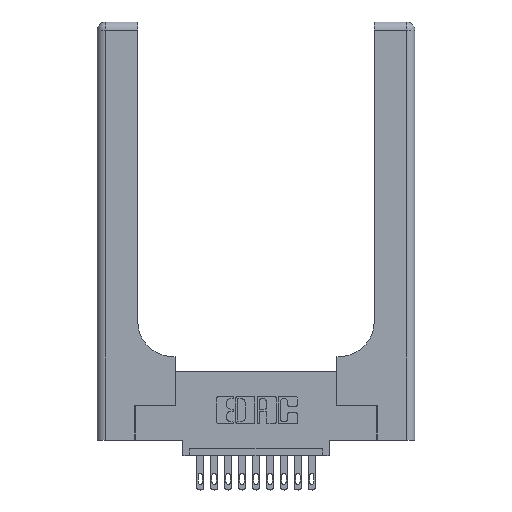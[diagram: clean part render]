
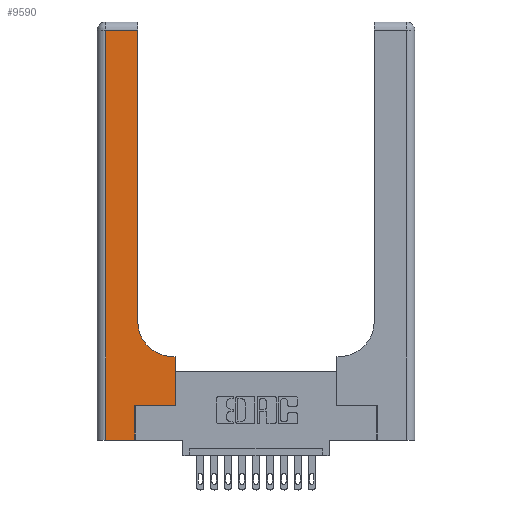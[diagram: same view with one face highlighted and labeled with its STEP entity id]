
A CAD part, top view. The second image highlights one B-rep face of the part: STEP entity #9590.
In plain terms, the highlighted planar face has unit normal (0, 0, 1).
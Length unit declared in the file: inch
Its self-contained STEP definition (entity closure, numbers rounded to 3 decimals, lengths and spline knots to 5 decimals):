
#40 = LINE ( 'NONE', #6423, #5369 ) ;
#183 = VERTEX_POINT ( 'NONE', #13133 ) ;
#448 = CARTESIAN_POINT ( 'NONE',  ( 0.06, 3., 0.37 ) ) ;
#511 = VERTEX_POINT ( 'NONE', #15085 ) ;
#565 = CARTESIAN_POINT ( 'NONE',  ( 0., 0., 0.37 ) ) ;
#735 = DIRECTION ( 'NONE',  ( 1., 0., 0. ) ) ;
#793 = EDGE_CURVE ( 'NONE', #9675, #12116, #40, .T. ) ;
#998 = CARTESIAN_POINT ( 'NONE',  ( 0., 2.94, 0.37 ) ) ;
#1002 = CARTESIAN_POINT ( 'NONE',  ( 0.5585, 0.25, 0.37 ) ) ;
#1090 = ORIENTED_EDGE ( 'NONE', *, *, #10468, .T. ) ;
#1092 = VECTOR ( 'NONE', #8857, 39.37008 ) ;
#1228 = CARTESIAN_POINT ( 'NONE',  ( 0.06, 0., 0.37 ) ) ;
#1243 = VERTEX_POINT ( 'NONE', #10867 ) ;
#2187 = VECTOR ( 'NONE', #735, 39.37008 ) ;
#2262 = CARTESIAN_POINT ( 'NONE',  ( 0.269, 0.25, 0.37 ) ) ;
#2326 = VECTOR ( 'NONE', #4971, 39.37008 ) ;
#2337 = DIRECTION ( 'NONE',  ( -1., 0., 0. ) ) ;
#2875 = CARTESIAN_POINT ( 'NONE',  ( 0.2915, 2.94, 0.37 ) ) ;
#3333 = ORIENTED_EDGE ( 'NONE', *, *, #13157, .T. ) ;
#3537 = DIRECTION ( 'NONE',  ( 0., 0., -1. ) ) ;
#3543 = EDGE_CURVE ( 'NONE', #9217, #9990, #8929, .T. ) ;
#4392 = ORIENTED_EDGE ( 'NONE', *, *, #7772, .T. ) ;
#4471 = CARTESIAN_POINT ( 'NONE',  ( 0., 3., 0.37 ) ) ;
#4577 = PLANE ( 'NONE',  #9491 ) ;
#4971 = DIRECTION ( 'NONE',  ( 0., 1., 0. ) ) ;
#4990 = ORIENTED_EDGE ( 'NONE', *, *, #11939, .T. ) ;
#4993 = CIRCLE ( 'NONE', #10254, 0.25 ) ;
#5369 = VECTOR ( 'NONE', #9749, 39.37008 ) ;
#5548 = LINE ( 'NONE', #998, #9497 ) ;
#5561 = LINE ( 'NONE', #565, #2187 ) ;
#5697 = LINE ( 'NONE', #1002, #2326 ) ;
#5817 = DIRECTION ( 'NONE',  ( 0., 0., -1. ) ) ;
#5955 = ORIENTED_EDGE ( 'NONE', *, *, #3543, .T. ) ;
#5991 = DIRECTION ( 'NONE',  ( -1., 0., 0. ) ) ;
#6092 = CARTESIAN_POINT ( 'NONE',  ( 0.269, 0., 0.37 ) ) ;
#6423 = CARTESIAN_POINT ( 'NONE',  ( 0.2915, 0.6, 0.37 ) ) ;
#6547 = CARTESIAN_POINT ( 'NONE',  ( 0.2915, 0.85, 0.37 ) ) ;
#6905 = CARTESIAN_POINT ( 'NONE',  ( 0.269, 0., 0.37 ) ) ;
#7039 = VERTEX_POINT ( 'NONE', #1228 ) ;
#7416 = LINE ( 'NONE', #448, #8202 ) ;
#7564 = VECTOR ( 'NONE', #13747, 39.37008 ) ;
#7772 = EDGE_CURVE ( 'NONE', #183, #1243, #8458, .T. ) ;
#7828 = FACE_OUTER_BOUND ( 'NONE', #9893, .T. ) ;
#8202 = VECTOR ( 'NONE', #10582, 39.37008 ) ;
#8458 = LINE ( 'NONE', #2262, #1092 ) ;
#8857 = DIRECTION ( 'NONE',  ( 1., 0., 0. ) ) ;
#8929 = LINE ( 'NONE', #15086, #7564 ) ;
#8968 = ORIENTED_EDGE ( 'NONE', *, *, #793, .T. ) ;
#9217 = VERTEX_POINT ( 'NONE', #6547 ) ;
#9491 = AXIS2_PLACEMENT_3D ( 'NONE', #4471, #5817, #5991 ) ;
#9497 = VECTOR ( 'NONE', #2337, 39.37008 ) ;
#9590 = ADVANCED_FACE ( 'NONE', ( #7828 ), #4577, .F. ) ;
#9675 = VERTEX_POINT ( 'NONE', #10587 ) ;
#9749 = DIRECTION ( 'NONE',  ( -1., 0., 0. ) ) ;
#9893 = EDGE_LOOP ( 'NONE', ( #5955, #3333, #1090, #14404, #4990, #4392, #12076, #8968, #10879 ) ) ;
#9896 = DIRECTION ( 'NONE',  ( 1., 0., 0. ) ) ;
#9950 = VECTOR ( 'NONE', #11904, 39.37008 ) ;
#9990 = VERTEX_POINT ( 'NONE', #2875 ) ;
#10254 = AXIS2_PLACEMENT_3D ( 'NONE', #12479, #3537, #9896 ) ;
#10468 = EDGE_CURVE ( 'NONE', #511, #7039, #7416, .T. ) ;
#10582 = DIRECTION ( 'NONE',  ( 0., -1., 0. ) ) ;
#10587 = CARTESIAN_POINT ( 'NONE',  ( 0.5585, 0.6, 0.37 ) ) ;
#10867 = CARTESIAN_POINT ( 'NONE',  ( 0.5585, 0.25, 0.37 ) ) ;
#10879 = ORIENTED_EDGE ( 'NONE', *, *, #10948, .T. ) ;
#10948 = EDGE_CURVE ( 'NONE', #12116, #9217, #4993, .T. ) ;
#11904 = DIRECTION ( 'NONE',  ( 0., 1., 0. ) ) ;
#11939 = EDGE_CURVE ( 'NONE', #16462, #183, #14769, .T. ) ;
#12076 = ORIENTED_EDGE ( 'NONE', *, *, #14996, .T. ) ;
#12116 = VERTEX_POINT ( 'NONE', #15088 ) ;
#12479 = CARTESIAN_POINT ( 'NONE',  ( 0.5415, 0.85, 0.37 ) ) ;
#13119 = EDGE_CURVE ( 'NONE', #7039, #16462, #5561, .T. ) ;
#13133 = CARTESIAN_POINT ( 'NONE',  ( 0.269, 0.25, 0.37 ) ) ;
#13157 = EDGE_CURVE ( 'NONE', #9990, #511, #5548, .T. ) ;
#13747 = DIRECTION ( 'NONE',  ( 0., 1., 0. ) ) ;
#14404 = ORIENTED_EDGE ( 'NONE', *, *, #13119, .T. ) ;
#14769 = LINE ( 'NONE', #6905, #9950 ) ;
#14996 = EDGE_CURVE ( 'NONE', #1243, #9675, #5697, .T. ) ;
#15085 = CARTESIAN_POINT ( 'NONE',  ( 0.06, 2.94, 0.37 ) ) ;
#15086 = CARTESIAN_POINT ( 'NONE',  ( 0.2915, 3., 0.37 ) ) ;
#15088 = CARTESIAN_POINT ( 'NONE',  ( 0.5415, 0.6, 0.37 ) ) ;
#16462 = VERTEX_POINT ( 'NONE', #6092 ) ;
